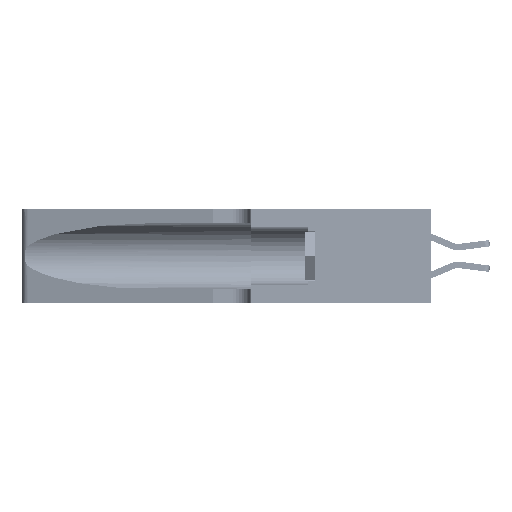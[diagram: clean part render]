
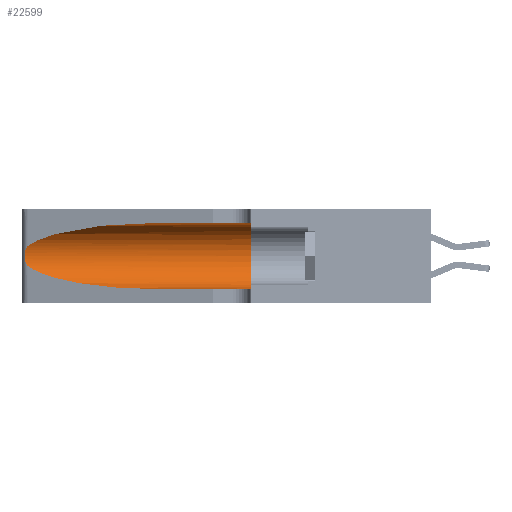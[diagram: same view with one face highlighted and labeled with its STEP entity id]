
A CAD part, left-side view. The second image highlights one B-rep face of the part: STEP entity #22599.
In plain terms, the highlighted cylindrical face has radius 3.308 mm (diameter 6.617 mm), a partial arc.
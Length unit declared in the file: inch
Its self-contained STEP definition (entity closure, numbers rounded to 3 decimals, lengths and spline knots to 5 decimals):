
#3126 = CARTESIAN_POINT ( 'NONE',  ( 0.2373, 1.15595, 0.08982 ) ) ;
#3546 = VECTOR ( 'NONE', #13957, 39.37008 ) ;
#3746 = CARTESIAN_POINT ( 'NONE',  ( 0.1305, 0.72297, 0.05475 ) ) ;
#4587 = CARTESIAN_POINT ( 'NONE',  ( 0.1305, 0.72297, 0.31525 ) ) ;
#4902 = CARTESIAN_POINT ( 'NONE',  ( 0.25639, 1.23184, 0.21858 ) ) ;
#5211 = VERTEX_POINT ( 'NONE', #17136 ) ;
#6765 = CARTESIAN_POINT ( 'NONE',  ( 0.25487, 1.22718, 0.14631 ) ) ;
#7586 = AXIS2_PLACEMENT_3D ( 'NONE', #31325, #9491, #35470 ) ;
#7800 = EDGE_LOOP ( 'NONE', ( #13663, #15812, #39516, #19297, #34785, #28005 ) ) ;
#8863 = CARTESIAN_POINT ( 'NONE',  ( 0.25555, 1.22994, 0.2215 ) ) ;
#9491 = DIRECTION ( 'NONE',  ( 0., 1., 0. ) ) ;
#9562 = DIRECTION ( 'NONE',  ( 0., -1., 0. ) ) ;
#11121 =( BOUNDED_CURVE ( )  B_SPLINE_CURVE ( 3, ( #6765, #3126, #39978, #3746 ),
 .UNSPECIFIED., .F., .T. ) 
 B_SPLINE_CURVE_WITH_KNOTS ( ( 4, 4 ),
 ( 3.44316, 4.71239 ),
 .UNSPECIFIED. ) 
 CURVE ( )  GEOMETRIC_REPRESENTATION_ITEM ( )  RATIONAL_B_SPLINE_CURVE ( ( 1., 0.87, 0.87, 1. ) ) 
 REPRESENTATION_ITEM ( '' )  );
#11743 = EDGE_CURVE ( 'NONE', #12880, #41568, #32826, .T. ) ;
#11922 = CARTESIAN_POINT ( 'NONE',  ( 0.2373, 1.15595, 0.28018 ) ) ;
#12541 = CARTESIAN_POINT ( 'NONE',  ( 0.25639, 1.23186, 0.15144 ) ) ;
#12577 =( BOUNDED_CURVE ( )  B_SPLINE_CURVE ( 3, ( #4587, #30094, #11922, #18445 ),
 .UNSPECIFIED., .F., .T. ) 
 B_SPLINE_CURVE_WITH_KNOTS ( ( 4, 4 ),
 ( 1.5708, 2.84003 ),
 .UNSPECIFIED. ) 
 CURVE ( )  GEOMETRIC_REPRESENTATION_ITEM ( )  RATIONAL_B_SPLINE_CURVE ( ( 1., 0.87, 0.87, 1. ) ) 
 REPRESENTATION_ITEM ( '' )  );
#12863 = CARTESIAN_POINT ( 'NONE',  ( 0.26018, 1.23835, 0.19895 ) ) ;
#12880 = VERTEX_POINT ( 'NONE', #39763 ) ;
#13663 = ORIENTED_EDGE ( 'NONE', *, *, #14387, .T. ) ;
#13957 = DIRECTION ( 'NONE',  ( 0., -1., 0. ) ) ;
#14387 = EDGE_CURVE ( 'NONE', #35784, #31372, #12577, .T. ) ;
#15812 = ORIENTED_EDGE ( 'NONE', *, *, #42877, .T. ) ;
#16077 = B_SPLINE_CURVE_WITH_KNOTS ( 'NONE', 3,
 ( #20005, #8863, #4902, #30547, #27202, #12863, #37749, #34390, #20173, #38232, #23830, #12541, #45475, #41765 ),
 .UNSPECIFIED., .F., .F.,
 ( 4, 2, 2, 2, 2, 2, 4 ),
 ( 0., 0.00027, 0.00053, 0.00107, 0.0016, 0.00187, 0.00214 ),
 .UNSPECIFIED. ) ;
#17136 = CARTESIAN_POINT ( 'NONE',  ( 0.1305, 0.35, 0.31525 ) ) ;
#18445 = CARTESIAN_POINT ( 'NONE',  ( 0.25487, 1.22718, 0.22369 ) ) ;
#18559 = CYLINDRICAL_SURFACE ( 'NONE', #28055, 0.13025 ) ;
#19246 = EDGE_CURVE ( 'NONE', #35784, #5211, #22902, .T. ) ;
#19297 = ORIENTED_EDGE ( 'NONE', *, *, #11743, .T. ) ;
#20005 = CARTESIAN_POINT ( 'NONE',  ( 0.25487, 1.22718, 0.22369 ) ) ;
#20173 = CARTESIAN_POINT ( 'NONE',  ( 0.26017, 1.23833, 0.17102 ) ) ;
#20702 = CARTESIAN_POINT ( 'NONE',  ( 0.25487, 1.22718, 0.14631 ) ) ;
#21712 = CARTESIAN_POINT ( 'NONE',  ( 0.1305, 1.61858, 0.31525 ) ) ;
#22599 = ADVANCED_FACE ( 'NONE', ( #29521 ), #18559, .F. ) ;
#22902 = LINE ( 'NONE', #21712, #3546 ) ;
#23279 = EDGE_CURVE ( 'NONE', #31655, #12880, #11121, .T. ) ;
#23830 = CARTESIAN_POINT ( 'NONE',  ( 0.25789, 1.23486, 0.15765 ) ) ;
#25304 = DIRECTION ( 'NONE',  ( 0., 0., -1. ) ) ;
#27202 = CARTESIAN_POINT ( 'NONE',  ( 0.25854, 1.2359, 0.20912 ) ) ;
#28005 = ORIENTED_EDGE ( 'NONE', *, *, #19246, .F. ) ;
#28055 = AXIS2_PLACEMENT_3D ( 'NONE', #32155, #28489, #25304 ) ;
#28489 = DIRECTION ( 'NONE',  ( 0., -1., 0. ) ) ;
#29521 = FACE_OUTER_BOUND ( 'NONE', #7800, .T. ) ;
#30094 = CARTESIAN_POINT ( 'NONE',  ( 0.18966, 0.96281, 0.31525 ) ) ;
#30547 = CARTESIAN_POINT ( 'NONE',  ( 0.25787, 1.23484, 0.2124 ) ) ;
#30978 = CARTESIAN_POINT ( 'NONE',  ( 0.1305, 0.35, 0.05475 ) ) ;
#31325 = CARTESIAN_POINT ( 'NONE',  ( 0.1305, 0.35, 0.185 ) ) ;
#31372 = VERTEX_POINT ( 'NONE', #40584 ) ;
#31655 = VERTEX_POINT ( 'NONE', #20702 ) ;
#32155 = CARTESIAN_POINT ( 'NONE',  ( 0.1305, 1.61858, 0.185 ) ) ;
#32826 = LINE ( 'NONE', #38948, #41455 ) ;
#34020 = CIRCLE ( 'NONE', #7586, 0.13025 ) ;
#34390 = CARTESIAN_POINT ( 'NONE',  ( 0.26075, 1.23896, 0.178 ) ) ;
#34785 = ORIENTED_EDGE ( 'NONE', *, *, #43031, .F. ) ;
#35470 = DIRECTION ( 'NONE',  ( 0., 0., 1. ) ) ;
#35784 = VERTEX_POINT ( 'NONE', #44051 ) ;
#37749 = CARTESIAN_POINT ( 'NONE',  ( 0.26075, 1.23896, 0.19203 ) ) ;
#38232 = CARTESIAN_POINT ( 'NONE',  ( 0.25856, 1.23593, 0.16098 ) ) ;
#38948 = CARTESIAN_POINT ( 'NONE',  ( 0.1305, 1.61858, 0.05475 ) ) ;
#39516 = ORIENTED_EDGE ( 'NONE', *, *, #23279, .T. ) ;
#39763 = CARTESIAN_POINT ( 'NONE',  ( 0.1305, 0.72297, 0.05475 ) ) ;
#39978 = CARTESIAN_POINT ( 'NONE',  ( 0.18966, 0.96281, 0.05475 ) ) ;
#40584 = CARTESIAN_POINT ( 'NONE',  ( 0.25487, 1.22718, 0.22369 ) ) ;
#41455 = VECTOR ( 'NONE', #9562, 39.37008 ) ;
#41568 = VERTEX_POINT ( 'NONE', #30978 ) ;
#41765 = CARTESIAN_POINT ( 'NONE',  ( 0.25487, 1.22718, 0.14631 ) ) ;
#42877 = EDGE_CURVE ( 'NONE', #31372, #31655, #16077, .T. ) ;
#43031 = EDGE_CURVE ( 'NONE', #5211, #41568, #34020, .T. ) ;
#44051 = CARTESIAN_POINT ( 'NONE',  ( 0.1305, 0.72297, 0.31525 ) ) ;
#45475 = CARTESIAN_POINT ( 'NONE',  ( 0.25555, 1.22993, 0.14849 ) ) ;
